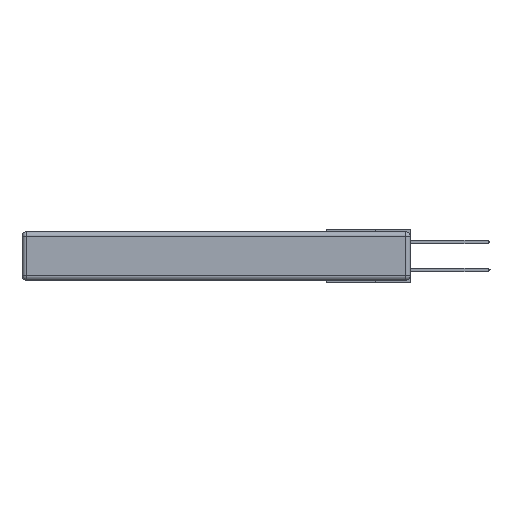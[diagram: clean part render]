
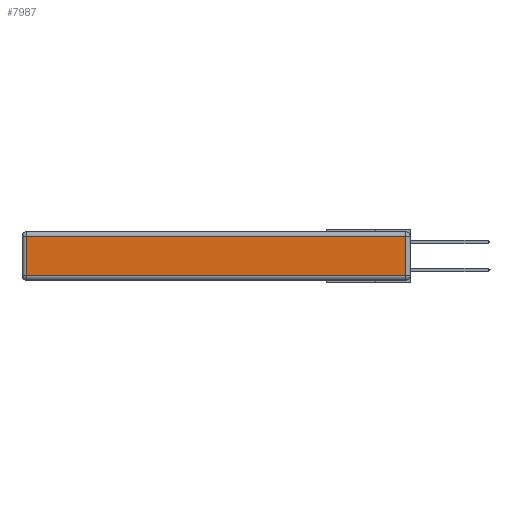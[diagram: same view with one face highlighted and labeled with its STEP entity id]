
A CAD part, left-side view. The second image highlights one B-rep face of the part: STEP entity #7987.
In plain terms, the highlighted planar face has unit normal (-1, 0, 0).
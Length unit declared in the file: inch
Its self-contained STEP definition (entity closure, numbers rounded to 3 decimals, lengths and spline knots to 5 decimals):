
#61 = CARTESIAN_POINT ( 'NONE',  ( 0., 0., -0.343 ) ) ;
#94 = VERTEX_POINT ( 'NONE', #13733 ) ;
#172 = CARTESIAN_POINT ( 'NONE',  ( 0., 2.75, -0.03 ) ) ;
#977 = ORIENTED_EDGE ( 'NONE', *, *, #11212, .T. ) ;
#1245 = EDGE_CURVE ( 'NONE', #8066, #3959, #5001, .T. ) ;
#1396 = EDGE_LOOP ( 'NONE', ( #977, #14826, #11014, #6839 ) ) ;
#1770 = DIRECTION ( 'NONE',  ( 0., -1., 0. ) ) ;
#2365 = CARTESIAN_POINT ( 'NONE',  ( 0., 0.03, -0.03 ) ) ;
#3959 = VERTEX_POINT ( 'NONE', #8534 ) ;
#4085 = CARTESIAN_POINT ( 'NONE',  ( 0., 0.03, -0.343 ) ) ;
#4087 = PLANE ( 'NONE',  #5537 ) ;
#4350 = VECTOR ( 'NONE', #7774, 39.37008 ) ;
#4946 = LINE ( 'NONE', #4085, #5804 ) ;
#5001 = LINE ( 'NONE', #11759, #4350 ) ;
#5193 = VECTOR ( 'NONE', #1770, 39.37008 ) ;
#5537 = AXIS2_PLACEMENT_3D ( 'NONE', #61, #16448, #17852 ) ;
#5580 = DIRECTION ( 'NONE',  ( 0., 1., 0. ) ) ;
#5804 = VECTOR ( 'NONE', #6664, 39.37008 ) ;
#6664 = DIRECTION ( 'NONE',  ( 0., 0., 1. ) ) ;
#6745 = VERTEX_POINT ( 'NONE', #2365 ) ;
#6839 = ORIENTED_EDGE ( 'NONE', *, *, #1245, .T. ) ;
#6925 = EDGE_CURVE ( 'NONE', #6745, #8066, #9701, .T. ) ;
#7469 = FACE_OUTER_BOUND ( 'NONE', #1396, .T. ) ;
#7774 = DIRECTION ( 'NONE',  ( 0., 0., -1. ) ) ;
#7987 = ADVANCED_FACE ( 'NONE', ( #7469 ), #4087, .T. ) ;
#8066 = VERTEX_POINT ( 'NONE', #15117 ) ;
#8534 = CARTESIAN_POINT ( 'NONE',  ( 0., 2.72, -0.313 ) ) ;
#9115 = LINE ( 'NONE', #14036, #5193 ) ;
#9701 = LINE ( 'NONE', #172, #12255 ) ;
#11014 = ORIENTED_EDGE ( 'NONE', *, *, #6925, .T. ) ;
#11212 = EDGE_CURVE ( 'NONE', #3959, #94, #9115, .T. ) ;
#11759 = CARTESIAN_POINT ( 'NONE',  ( 0., 2.72, -0.343 ) ) ;
#12255 = VECTOR ( 'NONE', #5580, 39.37008 ) ;
#13665 = EDGE_CURVE ( 'NONE', #94, #6745, #4946, .T. ) ;
#13733 = CARTESIAN_POINT ( 'NONE',  ( 0., 0.03, -0.313 ) ) ;
#14036 = CARTESIAN_POINT ( 'NONE',  ( 0., 0., -0.313 ) ) ;
#14826 = ORIENTED_EDGE ( 'NONE', *, *, #13665, .T. ) ;
#15117 = CARTESIAN_POINT ( 'NONE',  ( 0., 2.72, -0.03 ) ) ;
#16448 = DIRECTION ( 'NONE',  ( -1., 0., 0. ) ) ;
#17852 = DIRECTION ( 'NONE',  ( 0., 0., 1. ) ) ;
